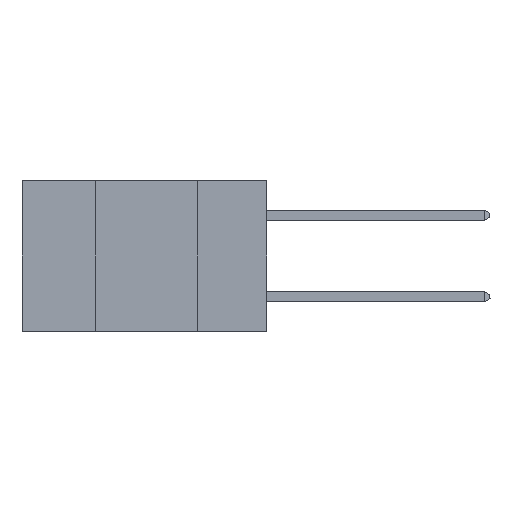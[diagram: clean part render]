
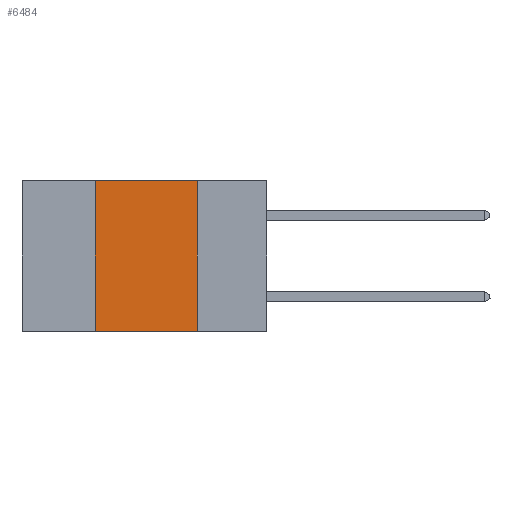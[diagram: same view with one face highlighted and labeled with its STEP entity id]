
A CAD part, left-side view. The second image highlights one B-rep face of the part: STEP entity #6484.
In plain terms, the highlighted planar face has unit normal (-1, 0, 0).
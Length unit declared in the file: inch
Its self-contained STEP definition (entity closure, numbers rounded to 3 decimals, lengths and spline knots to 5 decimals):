
#346 = DIRECTION ( 'NONE',  ( 0., 0., 1. ) ) ;
#1134 = DIRECTION ( 'NONE',  ( 1., 0., 0. ) ) ;
#1137 = CARTESIAN_POINT ( 'NONE',  ( 0., 0.6, 0. ) ) ;
#2078 = VECTOR ( 'NONE', #9236, 39.37008 ) ;
#2110 = FACE_OUTER_BOUND ( 'NONE', #26121, .T. ) ;
#3163 = ORIENTED_EDGE ( 'NONE', *, *, #25475, .F. ) ;
#4046 = LINE ( 'NONE', #5726, #16275 ) ;
#4399 = CARTESIAN_POINT ( 'NONE',  ( 0., 0.42, 0. ) ) ;
#4964 = VERTEX_POINT ( 'NONE', #13938 ) ;
#5520 = CARTESIAN_POINT ( 'NONE',  ( 0., 0.17, 0. ) ) ;
#5726 = CARTESIAN_POINT ( 'NONE',  ( 0., 0.17, 0. ) ) ;
#6484 = ADVANCED_FACE ( 'NONE', ( #2110 ), #21467, .F. ) ;
#6595 = VERTEX_POINT ( 'NONE', #5520 ) ;
#8089 = VECTOR ( 'NONE', #11921, 39.37008 ) ;
#9236 = DIRECTION ( 'NONE',  ( 0., -1., 0. ) ) ;
#9499 = LINE ( 'NONE', #4399, #9803 ) ;
#9803 = VECTOR ( 'NONE', #346, 39.37008 ) ;
#10134 = CARTESIAN_POINT ( 'NONE',  ( 0., 0.42, -0.37 ) ) ;
#11921 = DIRECTION ( 'NONE',  ( 0., -1., 0. ) ) ;
#13100 = EDGE_CURVE ( 'NONE', #24198, #4964, #9499, .T. ) ;
#13938 = CARTESIAN_POINT ( 'NONE',  ( 0., 0.42, 0. ) ) ;
#14075 = AXIS2_PLACEMENT_3D ( 'NONE', #17500, #1134, #21732 ) ;
#14321 = LINE ( 'NONE', #1137, #2078 ) ;
#16275 = VECTOR ( 'NONE', #20148, 39.37008 ) ;
#17243 = CARTESIAN_POINT ( 'NONE',  ( 0., 0.17, -0.37 ) ) ;
#17500 = CARTESIAN_POINT ( 'NONE',  ( 0., 0.6, 0. ) ) ;
#19986 = CARTESIAN_POINT ( 'NONE',  ( 0., 0.6, -0.37 ) ) ;
#20148 = DIRECTION ( 'NONE',  ( 0., 0., -1. ) ) ;
#20888 = ORIENTED_EDGE ( 'NONE', *, *, #26277, .T. ) ;
#21467 = PLANE ( 'NONE',  #14075 ) ;
#21732 = DIRECTION ( 'NONE',  ( 0., 0., -1. ) ) ;
#22020 = VERTEX_POINT ( 'NONE', #17243 ) ;
#22413 = ORIENTED_EDGE ( 'NONE', *, *, #23429, .F. ) ;
#22943 = LINE ( 'NONE', #19986, #8089 ) ;
#23429 = EDGE_CURVE ( 'NONE', #6595, #22020, #4046, .T. ) ;
#24198 = VERTEX_POINT ( 'NONE', #10134 ) ;
#25256 = ORIENTED_EDGE ( 'NONE', *, *, #13100, .F. ) ;
#25475 = EDGE_CURVE ( 'NONE', #4964, #6595, #14321, .T. ) ;
#26121 = EDGE_LOOP ( 'NONE', ( #22413, #3163, #25256, #20888 ) ) ;
#26277 = EDGE_CURVE ( 'NONE', #24198, #22020, #22943, .T. ) ;
